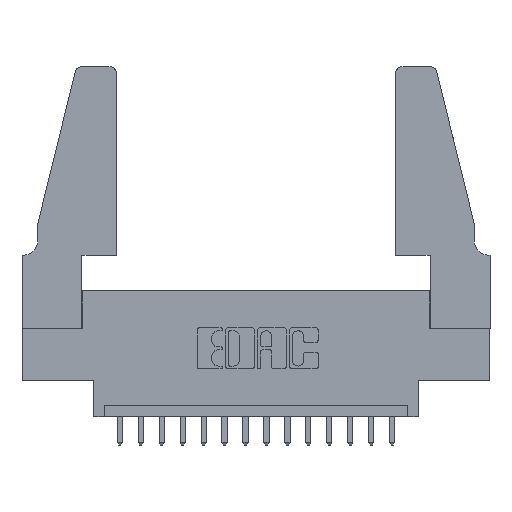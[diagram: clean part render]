
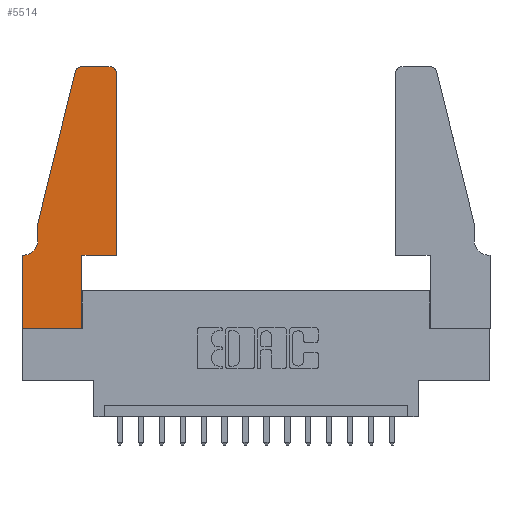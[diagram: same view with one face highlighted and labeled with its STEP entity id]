
A CAD part, top view. The second image highlights one B-rep face of the part: STEP entity #5514.
In plain terms, the highlighted planar face has unit normal (0, 0, 1).
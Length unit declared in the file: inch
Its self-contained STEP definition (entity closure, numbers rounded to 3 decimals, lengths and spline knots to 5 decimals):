
#20 = DIRECTION ( 'NONE',  ( 0., 1., 0. ) ) ;
#86 = VERTEX_POINT ( 'NONE', #8334 ) ;
#127 = VECTOR ( 'NONE', #14952, 39.37008 ) ;
#295 = CARTESIAN_POINT ( 'NONE',  ( 0.2605, 1.25, 0.37 ) ) ;
#376 = LINE ( 'NONE', #834, #13627 ) ;
#435 = DIRECTION ( 'NONE',  ( 0., 0., -1. ) ) ;
#444 = CARTESIAN_POINT ( 'NONE',  ( 0.0755, 0.5, 0.37 ) ) ;
#456 = FACE_OUTER_BOUND ( 'NONE', #1273, .T. ) ;
#479 = EDGE_CURVE ( 'NONE', #10701, #8952, #5273, .T. ) ;
#504 = ORIENTED_EDGE ( 'NONE', *, *, #9513, .T. ) ;
#711 = CARTESIAN_POINT ( 'NONE',  ( 0.4205, 1.22, 0.37 ) ) ;
#834 = CARTESIAN_POINT ( 'NONE',  ( 0.0755, 0.35, 0.37 ) ) ;
#1273 = EDGE_LOOP ( 'NONE', ( #504, #3388, #4415, #15183, #16583, #7337, #7768, #2000, #10909, #15620, #14573, #11191 ) ) ;
#1357 = AXIS2_PLACEMENT_3D ( 'NONE', #6835, #1739, #10649 ) ;
#1390 = CARTESIAN_POINT ( 'NONE',  ( 0.0055, 0.35, 0.37 ) ) ;
#1556 = EDGE_CURVE ( 'NONE', #86, #11653, #8985, .T. ) ;
#1651 = AXIS2_PLACEMENT_3D ( 'NONE', #10228, #3866, #2888 ) ;
#1732 = LINE ( 'NONE', #14900, #127 ) ;
#1739 = DIRECTION ( 'NONE',  ( 0., 0., 1. ) ) ;
#2000 = ORIENTED_EDGE ( 'NONE', *, *, #11075, .T. ) ;
#2101 = AXIS2_PLACEMENT_3D ( 'NONE', #711, #10975, #10344 ) ;
#2418 = VECTOR ( 'NONE', #7690, 39.37008 ) ;
#2655 = DIRECTION ( 'NONE',  ( -1., 0., 0. ) ) ;
#2888 = DIRECTION ( 'NONE',  ( 1., 0., 0. ) ) ;
#2965 = EDGE_CURVE ( 'NONE', #12827, #15330, #16405, .T. ) ;
#3191 = CIRCLE ( 'NONE', #4218, 0.07 ) ;
#3388 = ORIENTED_EDGE ( 'NONE', *, *, #1556, .T. ) ;
#3638 = CARTESIAN_POINT ( 'NONE',  ( 0., 0., 0.37 ) ) ;
#3801 = VERTEX_POINT ( 'NONE', #9327 ) ;
#3866 = DIRECTION ( 'NONE',  ( 0., 0., 1. ) ) ;
#3898 = PLANE ( 'NONE',  #1357 ) ;
#4041 = VECTOR ( 'NONE', #4868, 39.37008 ) ;
#4059 = VECTOR ( 'NONE', #20, 39.37008 ) ;
#4064 = VECTOR ( 'NONE', #2655, 39.37008 ) ;
#4218 = AXIS2_PLACEMENT_3D ( 'NONE', #6823, #435, #15851 ) ;
#4415 = ORIENTED_EDGE ( 'NONE', *, *, #7413, .T. ) ;
#4868 = DIRECTION ( 'NONE',  ( 1., 0., 0. ) ) ;
#5273 = LINE ( 'NONE', #9044, #4059 ) ;
#5514 = ADVANCED_FACE ( 'NONE', ( #456 ), #3898, .T. ) ;
#5735 = VERTEX_POINT ( 'NONE', #7217 ) ;
#5769 = EDGE_CURVE ( 'NONE', #13852, #9201, #376, .T. ) ;
#5792 = CARTESIAN_POINT ( 'NONE',  ( 0.0755, 0.5, 0.37 ) ) ;
#5994 = DIRECTION ( 'NONE',  ( 0., 1., 0. ) ) ;
#6009 = VECTOR ( 'NONE', #11006, 39.37008 ) ;
#6457 = LINE ( 'NONE', #295, #4064 ) ;
#6811 = VECTOR ( 'NONE', #5994, 39.37008 ) ;
#6823 = CARTESIAN_POINT ( 'NONE',  ( 0.0055, 0.42, 0.37 ) ) ;
#6835 = CARTESIAN_POINT ( 'NONE',  ( 0., 0.35, 0.37 ) ) ;
#7149 = CARTESIAN_POINT ( 'NONE',  ( 0.4505, 0.35, 0.37 ) ) ;
#7150 = EDGE_CURVE ( 'NONE', #9201, #3801, #1732, .T. ) ;
#7217 = CARTESIAN_POINT ( 'NONE',  ( 0.0755, 0.42, 0.37 ) ) ;
#7337 = ORIENTED_EDGE ( 'NONE', *, *, #5769, .T. ) ;
#7413 = EDGE_CURVE ( 'NONE', #11653, #16475, #16167, .T. ) ;
#7522 = VECTOR ( 'NONE', #15748, 39.37008 ) ;
#7690 = DIRECTION ( 'NONE',  ( 1., 0., 0. ) ) ;
#7768 = ORIENTED_EDGE ( 'NONE', *, *, #7150, .T. ) ;
#7795 = CARTESIAN_POINT ( 'NONE',  ( 0.4505, 0.35, 0.37 ) ) ;
#8334 = CARTESIAN_POINT ( 'NONE',  ( 0.284, 1.25, 0.37 ) ) ;
#8952 = VERTEX_POINT ( 'NONE', #14874 ) ;
#8985 = CIRCLE ( 'NONE', #1651, 0.03 ) ;
#9044 = CARTESIAN_POINT ( 'NONE',  ( 0.2865, 0.35, 0.37 ) ) ;
#9201 = VERTEX_POINT ( 'NONE', #12082 ) ;
#9327 = CARTESIAN_POINT ( 'NONE',  ( 0., 0., 0.37 ) ) ;
#9376 = LINE ( 'NONE', #5792, #6009 ) ;
#9513 = EDGE_CURVE ( 'NONE', #15330, #86, #6457, .T. ) ;
#10228 = CARTESIAN_POINT ( 'NONE',  ( 0.284, 1.22, 0.37 ) ) ;
#10344 = DIRECTION ( 'NONE',  ( 1., 0., 0. ) ) ;
#10480 = VERTEX_POINT ( 'NONE', #11491 ) ;
#10518 = EDGE_CURVE ( 'NONE', #8952, #10480, #11051, .T. ) ;
#10551 = CARTESIAN_POINT ( 'NONE',  ( 0.0755, 0.5, 0.37 ) ) ;
#10649 = DIRECTION ( 'NONE',  ( 1., 0., 0. ) ) ;
#10663 = EDGE_CURVE ( 'NONE', #5735, #13852, #3191, .T. ) ;
#10701 = VERTEX_POINT ( 'NONE', #16138 ) ;
#10760 = EDGE_CURVE ( 'NONE', #10480, #12827, #11636, .T. ) ;
#10859 = CARTESIAN_POINT ( 'NONE',  ( 0.4205, 1.25, 0.37 ) ) ;
#10909 = ORIENTED_EDGE ( 'NONE', *, *, #479, .T. ) ;
#10975 = DIRECTION ( 'NONE',  ( 0., 0., 1. ) ) ;
#11006 = DIRECTION ( 'NONE',  ( 0., -1., 0. ) ) ;
#11051 = LINE ( 'NONE', #7795, #2418 ) ;
#11075 = EDGE_CURVE ( 'NONE', #3801, #10701, #14838, .T. ) ;
#11168 = DIRECTION ( 'NONE',  ( -1., 0., 0. ) ) ;
#11191 = ORIENTED_EDGE ( 'NONE', *, *, #2965, .T. ) ;
#11491 = CARTESIAN_POINT ( 'NONE',  ( 0.4505, 0.35, 0.37 ) ) ;
#11636 = LINE ( 'NONE', #7149, #6811 ) ;
#11653 = VERTEX_POINT ( 'NONE', #15270 ) ;
#11799 = EDGE_CURVE ( 'NONE', #16475, #5735, #9376, .T. ) ;
#12082 = CARTESIAN_POINT ( 'NONE',  ( 0., 0.35, 0.37 ) ) ;
#12827 = VERTEX_POINT ( 'NONE', #15189 ) ;
#13627 = VECTOR ( 'NONE', #11168, 39.37008 ) ;
#13852 = VERTEX_POINT ( 'NONE', #1390 ) ;
#14573 = ORIENTED_EDGE ( 'NONE', *, *, #10760, .T. ) ;
#14838 = LINE ( 'NONE', #3638, #4041 ) ;
#14874 = CARTESIAN_POINT ( 'NONE',  ( 0.2865, 0.35, 0.37 ) ) ;
#14900 = CARTESIAN_POINT ( 'NONE',  ( 0., 0., 0.37 ) ) ;
#14952 = DIRECTION ( 'NONE',  ( 0., -1., 0. ) ) ;
#15183 = ORIENTED_EDGE ( 'NONE', *, *, #11799, .T. ) ;
#15189 = CARTESIAN_POINT ( 'NONE',  ( 0.4505, 1.22, 0.37 ) ) ;
#15270 = CARTESIAN_POINT ( 'NONE',  ( 0.25487, 1.22718, 0.37 ) ) ;
#15330 = VERTEX_POINT ( 'NONE', #10859 ) ;
#15620 = ORIENTED_EDGE ( 'NONE', *, *, #10518, .T. ) ;
#15748 = DIRECTION ( 'NONE',  ( -0.239, -0.971, 0. ) ) ;
#15851 = DIRECTION ( 'NONE',  ( -1., 0., 0. ) ) ;
#16138 = CARTESIAN_POINT ( 'NONE',  ( 0.2865, 0., 0.37 ) ) ;
#16167 = LINE ( 'NONE', #444, #7522 ) ;
#16405 = CIRCLE ( 'NONE', #2101, 0.03 ) ;
#16475 = VERTEX_POINT ( 'NONE', #10551 ) ;
#16583 = ORIENTED_EDGE ( 'NONE', *, *, #10663, .T. ) ;
